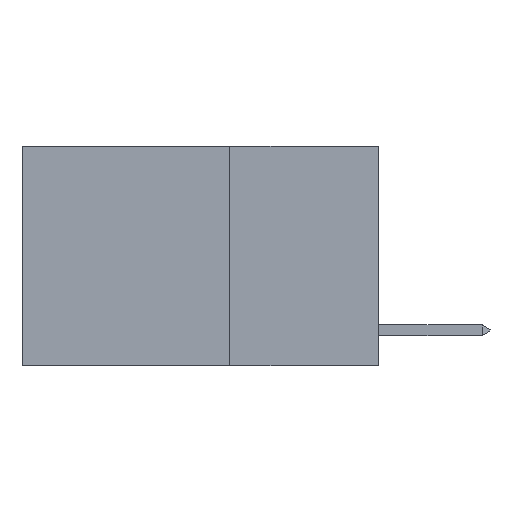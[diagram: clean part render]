
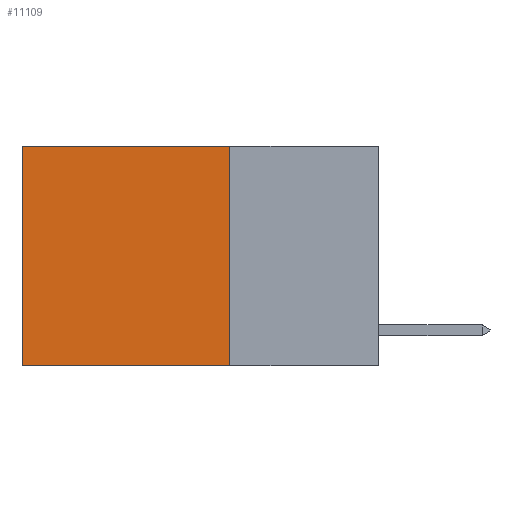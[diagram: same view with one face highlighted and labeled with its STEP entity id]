
A CAD part, left-side view. The second image highlights one B-rep face of the part: STEP entity #11109.
In plain terms, the highlighted planar face has unit normal (-1, 0, 0).
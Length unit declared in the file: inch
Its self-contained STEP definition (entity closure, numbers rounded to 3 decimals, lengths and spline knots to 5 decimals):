
#211 = DIRECTION ( 'NONE',  ( 0., 1., 0. ) ) ;
#302 = ORIENTED_EDGE ( 'NONE', *, *, #8191, .F. ) ;
#1548 = VERTEX_POINT ( 'NONE', #8388 ) ;
#2153 = VECTOR ( 'NONE', #6819, 39.37008 ) ;
#2349 = DIRECTION ( 'NONE',  ( 0., 0., -1. ) ) ;
#2709 = VERTEX_POINT ( 'NONE', #22819 ) ;
#2899 = CARTESIAN_POINT ( 'NONE',  ( 0.2625, 0.25, 0. ) ) ;
#3217 = VECTOR ( 'NONE', #6279, 39.37008 ) ;
#4537 = LINE ( 'NONE', #23101, #14111 ) ;
#4749 = ORIENTED_EDGE ( 'NONE', *, *, #21333, .F. ) ;
#4896 = DIRECTION ( 'NONE',  ( 0., 0., -1. ) ) ;
#5499 = VERTEX_POINT ( 'NONE', #10955 ) ;
#6020 = FACE_OUTER_BOUND ( 'NONE', #23777, .T. ) ;
#6279 = DIRECTION ( 'NONE',  ( 0., 0., -1. ) ) ;
#6819 = DIRECTION ( 'NONE',  ( 0., 1., 0. ) ) ;
#8131 = PLANE ( 'NONE',  #13945 ) ;
#8191 = EDGE_CURVE ( 'NONE', #5499, #1548, #17413, .T. ) ;
#8388 = CARTESIAN_POINT ( 'NONE',  ( 0.2625, 0.6, -0.37 ) ) ;
#10955 = CARTESIAN_POINT ( 'NONE',  ( 0.2625, 0.25, -0.37 ) ) ;
#11109 = ADVANCED_FACE ( 'NONE', ( #6020 ), #8131, .F. ) ;
#11111 = ORIENTED_EDGE ( 'NONE', *, *, #16397, .T. ) ;
#12273 = LINE ( 'NONE', #19506, #3217 ) ;
#13880 = DIRECTION ( 'NONE',  ( 1., 0., 0. ) ) ;
#13945 = AXIS2_PLACEMENT_3D ( 'NONE', #15602, #13880, #2349 ) ;
#13952 = LINE ( 'NONE', #2899, #18935 ) ;
#14111 = VECTOR ( 'NONE', #211, 39.37008 ) ;
#15011 = EDGE_CURVE ( 'NONE', #16681, #2709, #4537, .T. ) ;
#15602 = CARTESIAN_POINT ( 'NONE',  ( 0.2625, 0.25, 0. ) ) ;
#16397 = EDGE_CURVE ( 'NONE', #2709, #1548, #12273, .T. ) ;
#16681 = VERTEX_POINT ( 'NONE', #24104 ) ;
#17413 = LINE ( 'NONE', #20027, #2153 ) ;
#18935 = VECTOR ( 'NONE', #4896, 39.37008 ) ;
#19506 = CARTESIAN_POINT ( 'NONE',  ( 0.2625, 0.6, 0. ) ) ;
#20027 = CARTESIAN_POINT ( 'NONE',  ( 0.2625, 0.25, -0.37 ) ) ;
#21333 = EDGE_CURVE ( 'NONE', #16681, #5499, #13952, .T. ) ;
#22819 = CARTESIAN_POINT ( 'NONE',  ( 0.2625, 0.6, 0. ) ) ;
#23101 = CARTESIAN_POINT ( 'NONE',  ( 0.2625, 0.25, 0. ) ) ;
#23777 = EDGE_LOOP ( 'NONE', ( #11111, #302, #4749, #24000 ) ) ;
#24000 = ORIENTED_EDGE ( 'NONE', *, *, #15011, .T. ) ;
#24104 = CARTESIAN_POINT ( 'NONE',  ( 0.2625, 0.25, 0. ) ) ;
